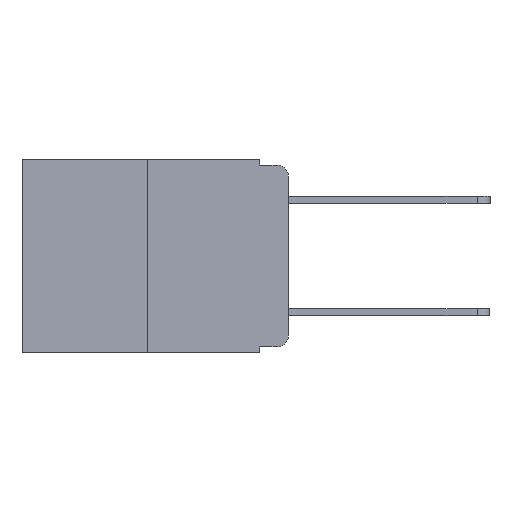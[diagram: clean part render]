
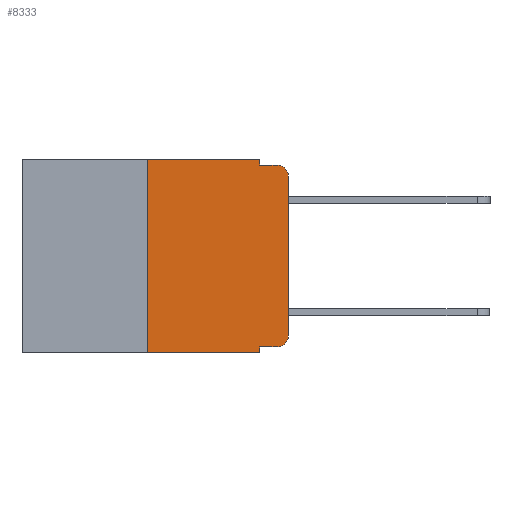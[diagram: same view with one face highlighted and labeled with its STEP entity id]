
A CAD part, left-side view. The second image highlights one B-rep face of the part: STEP entity #8333.
In plain terms, the highlighted planar face has unit normal (-1, 0, 0).
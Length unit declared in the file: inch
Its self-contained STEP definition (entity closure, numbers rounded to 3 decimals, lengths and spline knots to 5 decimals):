
#61 = DIRECTION ( 'NONE',  ( 0., 0., 1. ) ) ;
#168 = CARTESIAN_POINT ( 'NONE',  ( 0., 0.051, 0. ) ) ;
#374 = EDGE_LOOP ( 'NONE', ( #3351, #10808, #3700, #4079, #11320, #1083, #9320, #1924, #2316, #7807 ) ) ;
#595 = AXIS2_PLACEMENT_3D ( 'NONE', #702, #8196, #2038 ) ;
#597 = CARTESIAN_POINT ( 'NONE',  ( 0., 0.25, -0.343 ) ) ;
#702 = CARTESIAN_POINT ( 'NONE',  ( 0., 0.02, -0.03 ) ) ;
#734 = DIRECTION ( 'NONE',  ( 0., -1., 0. ) ) ;
#995 = LINE ( 'NONE', #9867, #6874 ) ;
#1083 = ORIENTED_EDGE ( 'NONE', *, *, #6205, .F. ) ;
#1200 = DIRECTION ( 'NONE',  ( 0., 0., -1. ) ) ;
#1241 = VERTEX_POINT ( 'NONE', #8902 ) ;
#1924 = ORIENTED_EDGE ( 'NONE', *, *, #5540, .F. ) ;
#2038 = DIRECTION ( 'NONE',  ( 0., 0., -1. ) ) ;
#2316 = ORIENTED_EDGE ( 'NONE', *, *, #4892, .T. ) ;
#2514 = CARTESIAN_POINT ( 'NONE',  ( 0., 0.051, -0.01 ) ) ;
#2905 = LINE ( 'NONE', #10192, #5398 ) ;
#3057 = FACE_OUTER_BOUND ( 'NONE', #374, .T. ) ;
#3224 = DIRECTION ( 'NONE',  ( 0., 0., -1. ) ) ;
#3234 = CARTESIAN_POINT ( 'NONE',  ( 0., 0.051, 0. ) ) ;
#3316 = CARTESIAN_POINT ( 'NONE',  ( 0., 0.02, -0.01 ) ) ;
#3351 = ORIENTED_EDGE ( 'NONE', *, *, #8651, .T. ) ;
#3478 = VERTEX_POINT ( 'NONE', #10230 ) ;
#3578 = PLANE ( 'NONE',  #9076 ) ;
#3700 = ORIENTED_EDGE ( 'NONE', *, *, #7457, .F. ) ;
#3791 = AXIS2_PLACEMENT_3D ( 'NONE', #12819, #7651, #1200 ) ;
#3965 = LINE ( 'NONE', #6870, #10993 ) ;
#3987 = CARTESIAN_POINT ( 'NONE',  ( 0., 0.02, -0.333 ) ) ;
#4079 = ORIENTED_EDGE ( 'NONE', *, *, #6827, .F. ) ;
#4276 = EDGE_CURVE ( 'NONE', #4560, #4514, #11782, .T. ) ;
#4407 = DIRECTION ( 'NONE',  ( 0., -1., 0. ) ) ;
#4451 = VECTOR ( 'NONE', #4407, 39.37008 ) ;
#4514 = VERTEX_POINT ( 'NONE', #5917 ) ;
#4560 = VERTEX_POINT ( 'NONE', #3987 ) ;
#4565 = VECTOR ( 'NONE', #8860, 39.37008 ) ;
#4892 = EDGE_CURVE ( 'NONE', #10944, #4560, #11376, .T. ) ;
#5046 = CARTESIAN_POINT ( 'NONE',  ( 0., 0.051, -0.343 ) ) ;
#5398 = VECTOR ( 'NONE', #11070, 39.37008 ) ;
#5493 = VECTOR ( 'NONE', #734, 39.37008 ) ;
#5540 = EDGE_CURVE ( 'NONE', #10944, #11571, #8119, .T. ) ;
#5616 = DIRECTION ( 'NONE',  ( 0., 0., -1. ) ) ;
#5753 = DIRECTION ( 'NONE',  ( 0., -1., 0. ) ) ;
#5847 = VERTEX_POINT ( 'NONE', #597 ) ;
#5917 = CARTESIAN_POINT ( 'NONE',  ( 0., 0., -0.313 ) ) ;
#6205 = EDGE_CURVE ( 'NONE', #5847, #3478, #2905, .T. ) ;
#6827 = EDGE_CURVE ( 'NONE', #9034, #9646, #995, .T. ) ;
#6870 = CARTESIAN_POINT ( 'NONE',  ( 0., 0., 0. ) ) ;
#6874 = VECTOR ( 'NONE', #3224, 39.37008 ) ;
#7011 = CIRCLE ( 'NONE', #595, 0.02 ) ;
#7328 = CARTESIAN_POINT ( 'NONE',  ( 0., 0.473, 0. ) ) ;
#7457 = EDGE_CURVE ( 'NONE', #9646, #11942, #12860, .T. ) ;
#7651 = DIRECTION ( 'NONE',  ( -1., 0., 0. ) ) ;
#7807 = ORIENTED_EDGE ( 'NONE', *, *, #4276, .T. ) ;
#7856 = DIRECTION ( 'NONE',  ( 0., 0., -1. ) ) ;
#7960 = CARTESIAN_POINT ( 'NONE',  ( 0., 0.473, -0.343 ) ) ;
#8050 = EDGE_CURVE ( 'NONE', #1241, #11942, #7011, .T. ) ;
#8119 = LINE ( 'NONE', #168, #9628 ) ;
#8196 = DIRECTION ( 'NONE',  ( -1., 0., 0. ) ) ;
#8278 = VECTOR ( 'NONE', #5753, 39.37008 ) ;
#8333 = ADVANCED_FACE ( 'NONE', ( #3057 ), #3578, .F. ) ;
#8651 = EDGE_CURVE ( 'NONE', #4514, #1241, #3965, .T. ) ;
#8671 = CARTESIAN_POINT ( 'NONE',  ( 0., 0.051, -0.333 ) ) ;
#8860 = DIRECTION ( 'NONE',  ( 0., -1., 0. ) ) ;
#8902 = CARTESIAN_POINT ( 'NONE',  ( 0., 0., -0.03 ) ) ;
#9034 = VERTEX_POINT ( 'NONE', #3234 ) ;
#9076 = AXIS2_PLACEMENT_3D ( 'NONE', #10970, #11001, #5616 ) ;
#9187 = EDGE_CURVE ( 'NONE', #3478, #9034, #10589, .T. ) ;
#9320 = ORIENTED_EDGE ( 'NONE', *, *, #11315, .T. ) ;
#9470 = LINE ( 'NONE', #7960, #4565 ) ;
#9628 = VECTOR ( 'NONE', #7856, 39.37008 ) ;
#9646 = VERTEX_POINT ( 'NONE', #2514 ) ;
#9867 = CARTESIAN_POINT ( 'NONE',  ( 0., 0.051, 0. ) ) ;
#9901 = CARTESIAN_POINT ( 'NONE',  ( 0., 0.051, -0.333 ) ) ;
#10192 = CARTESIAN_POINT ( 'NONE',  ( 0., 0.25, 0. ) ) ;
#10230 = CARTESIAN_POINT ( 'NONE',  ( 0., 0.25, 0. ) ) ;
#10262 = CARTESIAN_POINT ( 'NONE',  ( 0., 0.051, -0.01 ) ) ;
#10589 = LINE ( 'NONE', #7328, #5493 ) ;
#10808 = ORIENTED_EDGE ( 'NONE', *, *, #8050, .T. ) ;
#10944 = VERTEX_POINT ( 'NONE', #8671 ) ;
#10970 = CARTESIAN_POINT ( 'NONE',  ( 0., 0.473, 0. ) ) ;
#10993 = VECTOR ( 'NONE', #61, 39.37008 ) ;
#11001 = DIRECTION ( 'NONE',  ( 1., 0., 0. ) ) ;
#11070 = DIRECTION ( 'NONE',  ( 0., 0., 1. ) ) ;
#11315 = EDGE_CURVE ( 'NONE', #5847, #11571, #9470, .T. ) ;
#11320 = ORIENTED_EDGE ( 'NONE', *, *, #9187, .F. ) ;
#11376 = LINE ( 'NONE', #9901, #4451 ) ;
#11571 = VERTEX_POINT ( 'NONE', #5046 ) ;
#11782 = CIRCLE ( 'NONE', #3791, 0.02 ) ;
#11942 = VERTEX_POINT ( 'NONE', #3316 ) ;
#12819 = CARTESIAN_POINT ( 'NONE',  ( 0., 0.02, -0.313 ) ) ;
#12860 = LINE ( 'NONE', #10262, #8278 ) ;
